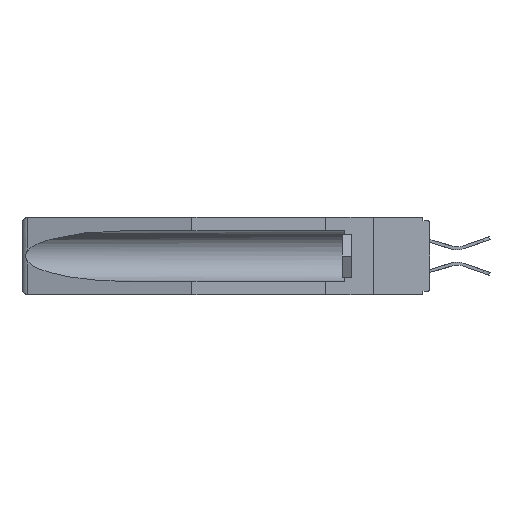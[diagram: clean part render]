
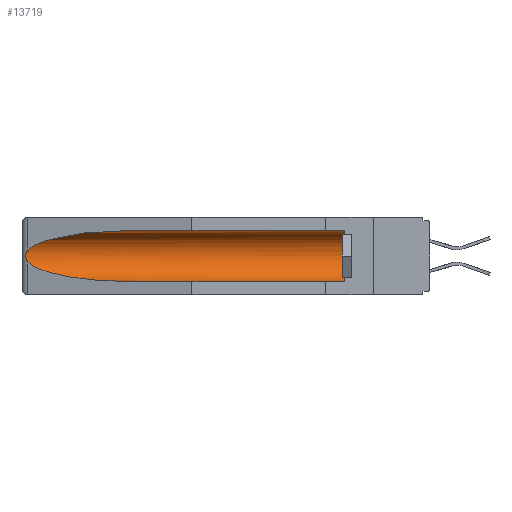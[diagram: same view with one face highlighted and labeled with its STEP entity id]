
A CAD part, left-side view. The second image highlights one B-rep face of the part: STEP entity #13719.
In plain terms, the highlighted cylindrical face has radius 2.857 mm (diameter 5.715 mm), a partial arc.
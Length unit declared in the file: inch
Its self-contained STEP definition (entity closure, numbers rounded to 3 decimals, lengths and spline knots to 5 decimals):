
#417 = CYLINDRICAL_SURFACE ( 'NONE', #16269, 0.1125 ) ;
#471 = EDGE_CURVE ( 'NONE', #3129, #17424, #10892, .T. ) ;
#503 = CARTESIAN_POINT ( 'NONE',  ( 0.2673, 1.53269, -0.17917 ) ) ;
#561 = CARTESIAN_POINT ( 'NONE',  ( 0.155, -0.30754, -0.059 ) ) ;
#681 = EDGE_CURVE ( 'NONE', #17424, #17878, #4911, .T. ) ;
#740 = EDGE_CURVE ( 'NONE', #17878, #22139, #21629, .T. ) ;
#1362 = CARTESIAN_POINT ( 'NONE',  ( 0.26537, 1.52718, -0.19328 ) ) ;
#2465 = CARTESIAN_POINT ( 'NONE',  ( 0.25451, 1.48313, -0.24835 ) ) ;
#2481 = CARTESIAN_POINT ( 'NONE',  ( 0.2673, 1.5327, -0.16383 ) ) ;
#2563 = CARTESIAN_POINT ( 'NONE',  ( 0.26654, 1.53092, -0.15636 ) ) ;
#3129 = VERTEX_POINT ( 'NONE', #11501 ) ;
#3672 = CARTESIAN_POINT ( 'NONE',  ( 0.155, 0.126, -0.1715 ) ) ;
#4911 = LINE ( 'NONE', #561, #14570 ) ;
#5483 = DIRECTION ( 'NONE',  ( 0., 0., 1. ) ) ;
#5521 = EDGE_CURVE ( 'NONE', #3129, #12574, #12276, .T. ) ;
#6027 = CARTESIAN_POINT ( 'NONE',  ( 0.155, 1.07973, -0.284 ) ) ;
#6045 = CARTESIAN_POINT ( 'NONE',  ( 0.2675, 1.53308, -0.16763 ) ) ;
#7280 = CARTESIAN_POINT ( 'NONE',  ( 0.155, 0.126, -0.059 ) ) ;
#7481 = CARTESIAN_POINT ( 'NONE',  ( 0.26537, 1.52718, -0.14972 ) ) ;
#7511 = CARTESIAN_POINT ( 'NONE',  ( 0.155, -0.30754, -0.1715 ) ) ;
#7554 = EDGE_CURVE ( 'NONE', #15991, #12574, #13096, .T. ) ;
#7997 = CARTESIAN_POINT ( 'NONE',  ( 0.26537, 1.52718, -0.14972 ) ) ;
#8673 = EDGE_CURVE ( 'NONE', #22139, #15991, #16398, .T. ) ;
#8995 = DIRECTION ( 'NONE',  ( 0., 1., 0. ) ) ;
#9309 = CARTESIAN_POINT ( 'NONE',  ( 0.26597, 1.52961, -0.15275 ) ) ;
#9612 = CARTESIAN_POINT ( 'NONE',  ( 0.26597, 1.5296, -0.19026 ) ) ;
#9840 = CARTESIAN_POINT ( 'NONE',  ( 0.26537, 1.52718, -0.19328 ) ) ;
#9923 = CARTESIAN_POINT ( 'NONE',  ( 0.25451, 1.48313, -0.09465 ) ) ;
#10402 = ORIENTED_EDGE ( 'NONE', *, *, #740, .T. ) ;
#10850 = VECTOR ( 'NONE', #8995, 39.37008 ) ;
#10892 = CIRCLE ( 'NONE', #21211, 0.1125 ) ;
#10964 = EDGE_LOOP ( 'NONE', ( #10402, #22398, #14163, #14711, #13996, #16893 ) ) ;
#10972 = CARTESIAN_POINT ( 'NONE',  ( 0.155, -0.30754, -0.284 ) ) ;
#11501 = CARTESIAN_POINT ( 'NONE',  ( 0.155, 0.126, -0.284 ) ) ;
#12276 = LINE ( 'NONE', #10972, #10850 ) ;
#12574 = VERTEX_POINT ( 'NONE', #6027 ) ;
#12611 = FACE_OUTER_BOUND ( 'NONE', #10964, .T. ) ;
#12635 = CARTESIAN_POINT ( 'NONE',  ( 0.155, 1.07973, -0.059 ) ) ;
#13096 =( BOUNDED_CURVE ( )  B_SPLINE_CURVE ( 3, ( #9840, #2465, #15201, #18967 ),
 .UNSPECIFIED., .F., .F. ) 
 B_SPLINE_CURVE_WITH_KNOTS ( ( 4, 4 ),
 ( 0.1948, 1.5708 ),
 .UNSPECIFIED. ) 
 CURVE ( )  GEOMETRIC_REPRESENTATION_ITEM ( )  RATIONAL_B_SPLINE_CURVE ( ( 1., 0.848, 0.848, 1. ) ) 
 REPRESENTATION_ITEM ( '' )  );
#13190 = CARTESIAN_POINT ( 'NONE',  ( 0.26655, 1.53094, -0.18657 ) ) ;
#13344 = CARTESIAN_POINT ( 'NONE',  ( 0.2675, 1.53308, -0.17534 ) ) ;
#13719 = ADVANCED_FACE ( 'NONE', ( #12611 ), #417, .F. ) ;
#13996 = ORIENTED_EDGE ( 'NONE', *, *, #471, .T. ) ;
#14163 = ORIENTED_EDGE ( 'NONE', *, *, #7554, .T. ) ;
#14570 = VECTOR ( 'NONE', #22616, 39.37008 ) ;
#14711 = ORIENTED_EDGE ( 'NONE', *, *, #5521, .F. ) ;
#15125 = DIRECTION ( 'NONE',  ( 0., 1., 0. ) ) ;
#15201 = CARTESIAN_POINT ( 'NONE',  ( 0.21114, 1.30732, -0.284 ) ) ;
#15294 = CARTESIAN_POINT ( 'NONE',  ( 0.26537, 1.52718, -0.19328 ) ) ;
#15434 = CARTESIAN_POINT ( 'NONE',  ( 0.26537, 1.52718, -0.14972 ) ) ;
#15991 = VERTEX_POINT ( 'NONE', #1362 ) ;
#16269 = AXIS2_PLACEMENT_3D ( 'NONE', #7511, #15125, #16891 ) ;
#16398 = B_SPLINE_CURVE_WITH_KNOTS ( 'NONE', 3,
 ( #7481, #9309, #2563, #2481, #6045, #13344, #503, #13190, #9612, #15294 ),
 .UNSPECIFIED., .F., .F.,
 ( 4, 2, 2, 2, 4 ),
 ( 0., 0.00029, 0.00058, 0.00087, 0.00117 ),
 .UNSPECIFIED. ) ;
#16418 = DIRECTION ( 'NONE',  ( 0., -1., 0. ) ) ;
#16891 = DIRECTION ( 'NONE',  ( 0., 0., 1. ) ) ;
#16893 = ORIENTED_EDGE ( 'NONE', *, *, #681, .T. ) ;
#17188 = CARTESIAN_POINT ( 'NONE',  ( 0.155, 1.07973, -0.059 ) ) ;
#17424 = VERTEX_POINT ( 'NONE', #7280 ) ;
#17878 = VERTEX_POINT ( 'NONE', #12635 ) ;
#18967 = CARTESIAN_POINT ( 'NONE',  ( 0.155, 1.07973, -0.284 ) ) ;
#19042 = CARTESIAN_POINT ( 'NONE',  ( 0.21114, 1.30732, -0.059 ) ) ;
#21211 = AXIS2_PLACEMENT_3D ( 'NONE', #3672, #16418, #5483 ) ;
#21629 =( BOUNDED_CURVE ( )  B_SPLINE_CURVE ( 3, ( #17188, #19042, #9923, #15434 ),
 .UNSPECIFIED., .F., .F. ) 
 B_SPLINE_CURVE_WITH_KNOTS ( ( 4, 4 ),
 ( 4.71239, 6.08839 ),
 .UNSPECIFIED. ) 
 CURVE ( )  GEOMETRIC_REPRESENTATION_ITEM ( )  RATIONAL_B_SPLINE_CURVE ( ( 1., 0.848, 0.848, 1. ) ) 
 REPRESENTATION_ITEM ( '' )  );
#22139 = VERTEX_POINT ( 'NONE', #7997 ) ;
#22398 = ORIENTED_EDGE ( 'NONE', *, *, #8673, .T. ) ;
#22616 = DIRECTION ( 'NONE',  ( 0., 1., 0. ) ) ;
